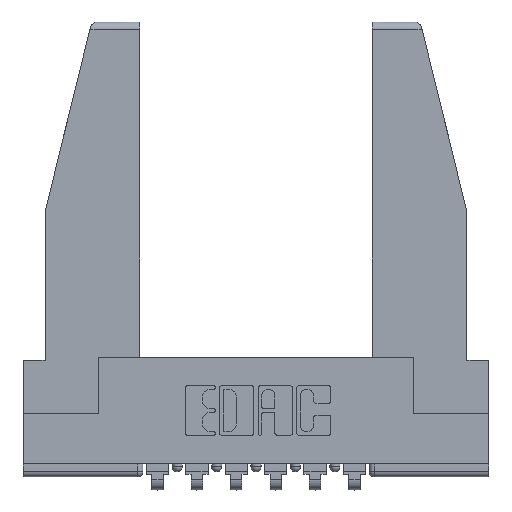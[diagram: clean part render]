
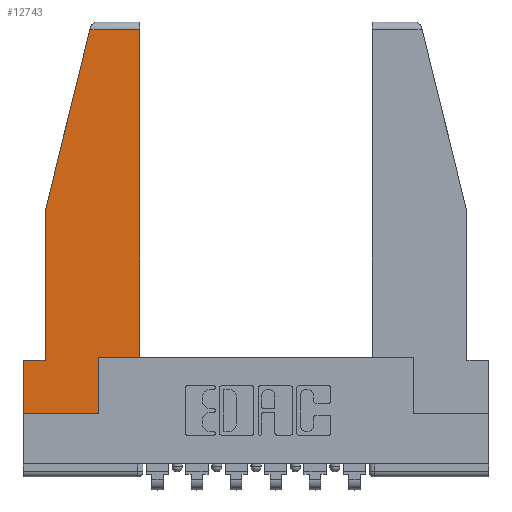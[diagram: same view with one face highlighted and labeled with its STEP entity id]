
A CAD part, top view. The second image highlights one B-rep face of the part: STEP entity #12743.
In plain terms, the highlighted planar face has unit normal (0, 0, 1).
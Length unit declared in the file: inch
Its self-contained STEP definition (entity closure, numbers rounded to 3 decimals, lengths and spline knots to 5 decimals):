
#192 = ORIENTED_EDGE ( 'NONE', *, *, #7958, .T. ) ;
#205 = DIRECTION ( 'NONE',  ( -1., 0., 0. ) ) ;
#227 = EDGE_CURVE ( 'NONE', #11809, #1380, #10423, .T. ) ;
#365 = CARTESIAN_POINT ( 'NONE',  ( 0., 0., 0. ) ) ;
#497 = CARTESIAN_POINT ( 'NONE',  ( 0., 0., 0. ) ) ;
#517 = CARTESIAN_POINT ( 'NONE',  ( 0., 0.21, 0. ) ) ;
#794 = DIRECTION ( 'NONE',  ( 1., 0., 0. ) ) ;
#1380 = VERTEX_POINT ( 'NONE', #3621 ) ;
#1431 = VECTOR ( 'NONE', #9479, 39.37008 ) ;
#1538 = VERTEX_POINT ( 'NONE', #4978 ) ;
#1564 = CARTESIAN_POINT ( 'NONE',  ( 0., 0.21, 0. ) ) ;
#1834 = VERTEX_POINT ( 'NONE', #4002 ) ;
#2245 = VERTEX_POINT ( 'NONE', #365 ) ;
#2507 = DIRECTION ( 'NONE',  ( 0., 0., 1. ) ) ;
#2600 = CARTESIAN_POINT ( 'NONE',  ( 0.461, 1.52, 0. ) ) ;
#2631 = EDGE_CURVE ( 'NONE', #11027, #6464, #4052, .T. ) ;
#2651 = LINE ( 'NONE', #8580, #5749 ) ;
#2909 = EDGE_CURVE ( 'NONE', #1380, #11027, #10781, .T. ) ;
#3002 = EDGE_CURVE ( 'NONE', #6464, #1834, #11641, .T. ) ;
#3395 = LINE ( 'NONE', #12476, #1431 ) ;
#3473 = ORIENTED_EDGE ( 'NONE', *, *, #2631, .T. ) ;
#3511 = EDGE_LOOP ( 'NONE', ( #3473, #6750, #9803, #192, #11223, #9784, #12626, #4335, #5338 ) ) ;
#3618 = DIRECTION ( 'NONE',  ( 1., 0., 0. ) ) ;
#3621 = CARTESIAN_POINT ( 'NONE',  ( 0.297, 0.223, 0. ) ) ;
#3668 = DIRECTION ( 'NONE',  ( 1., 0., 0. ) ) ;
#3799 = LINE ( 'NONE', #6682, #9373 ) ;
#4002 = CARTESIAN_POINT ( 'NONE',  ( 0.2636, 1.52, 0. ) ) ;
#4052 = LINE ( 'NONE', #7981, #10561 ) ;
#4335 = ORIENTED_EDGE ( 'NONE', *, *, #227, .T. ) ;
#4358 = CARTESIAN_POINT ( 'NONE',  ( 0.297, 0., 0. ) ) ;
#4491 = CARTESIAN_POINT ( 'NONE',  ( 0.297, 0., 0. ) ) ;
#4837 = CARTESIAN_POINT ( 'NONE',  ( 0.297, 0.223, 0. ) ) ;
#4978 = CARTESIAN_POINT ( 'NONE',  ( 0.086, 0.21, 0. ) ) ;
#5058 = CARTESIAN_POINT ( 'NONE',  ( 0.086, 0.8, 0. ) ) ;
#5120 = EDGE_CURVE ( 'NONE', #1538, #11944, #7744, .T. ) ;
#5338 = ORIENTED_EDGE ( 'NONE', *, *, #2909, .T. ) ;
#5749 = VECTOR ( 'NONE', #12568, 39.37008 ) ;
#5927 = VECTOR ( 'NONE', #9524, 39.37008 ) ;
#6292 = EDGE_CURVE ( 'NONE', #11944, #2245, #7437, .T. ) ;
#6464 = VERTEX_POINT ( 'NONE', #2600 ) ;
#6682 = CARTESIAN_POINT ( 'NONE',  ( 0., 0., 0. ) ) ;
#6750 = ORIENTED_EDGE ( 'NONE', *, *, #3002, .T. ) ;
#6785 = VECTOR ( 'NONE', #205, 39.37008 ) ;
#7125 = EDGE_CURVE ( 'NONE', #1834, #11419, #2651, .T. ) ;
#7437 = LINE ( 'NONE', #517, #5927 ) ;
#7602 = VECTOR ( 'NONE', #11706, 39.37008 ) ;
#7719 = CARTESIAN_POINT ( 'NONE',  ( 0., 1.52, 0. ) ) ;
#7744 = LINE ( 'NONE', #11727, #6785 ) ;
#7958 = EDGE_CURVE ( 'NONE', #11419, #1538, #3395, .T. ) ;
#7981 = CARTESIAN_POINT ( 'NONE',  ( 0.461, 0.223, 0. ) ) ;
#8576 = FACE_OUTER_BOUND ( 'NONE', #3511, .T. ) ;
#8580 = CARTESIAN_POINT ( 'NONE',  ( 0.271, 1.55, 0. ) ) ;
#8838 = VECTOR ( 'NONE', #794, 39.37008 ) ;
#9208 = AXIS2_PLACEMENT_3D ( 'NONE', #497, #2507, #3618 ) ;
#9373 = VECTOR ( 'NONE', #3668, 39.37008 ) ;
#9479 = DIRECTION ( 'NONE',  ( 0., -1., 0. ) ) ;
#9524 = DIRECTION ( 'NONE',  ( 0., -1., 0. ) ) ;
#9784 = ORIENTED_EDGE ( 'NONE', *, *, #6292, .T. ) ;
#9803 = ORIENTED_EDGE ( 'NONE', *, *, #7125, .T. ) ;
#10423 = LINE ( 'NONE', #4491, #11856 ) ;
#10561 = VECTOR ( 'NONE', #10982, 39.37008 ) ;
#10693 = EDGE_CURVE ( 'NONE', #2245, #11809, #3799, .T. ) ;
#10781 = LINE ( 'NONE', #4837, #8838 ) ;
#10982 = DIRECTION ( 'NONE',  ( 0., 1., 0. ) ) ;
#11027 = VERTEX_POINT ( 'NONE', #11077 ) ;
#11077 = CARTESIAN_POINT ( 'NONE',  ( 0.461, 0.223, 0. ) ) ;
#11223 = ORIENTED_EDGE ( 'NONE', *, *, #5120, .T. ) ;
#11419 = VERTEX_POINT ( 'NONE', #5058 ) ;
#11641 = LINE ( 'NONE', #7719, #7602 ) ;
#11706 = DIRECTION ( 'NONE',  ( -1., 0., 0. ) ) ;
#11727 = CARTESIAN_POINT ( 'NONE',  ( 0., 0.21, 0. ) ) ;
#11809 = VERTEX_POINT ( 'NONE', #4358 ) ;
#11856 = VECTOR ( 'NONE', #12523, 39.37008 ) ;
#11944 = VERTEX_POINT ( 'NONE', #1564 ) ;
#12476 = CARTESIAN_POINT ( 'NONE',  ( 0.086, 0.8, 0. ) ) ;
#12523 = DIRECTION ( 'NONE',  ( 0., 1., 0. ) ) ;
#12561 = PLANE ( 'NONE',  #9208 ) ;
#12568 = DIRECTION ( 'NONE',  ( -0.239, -0.971, 0. ) ) ;
#12626 = ORIENTED_EDGE ( 'NONE', *, *, #10693, .T. ) ;
#12743 = ADVANCED_FACE ( 'NONE', ( #8576 ), #12561, .T. ) ;
